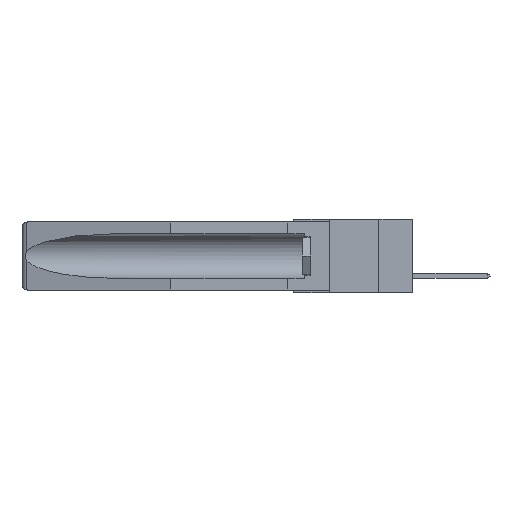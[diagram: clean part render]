
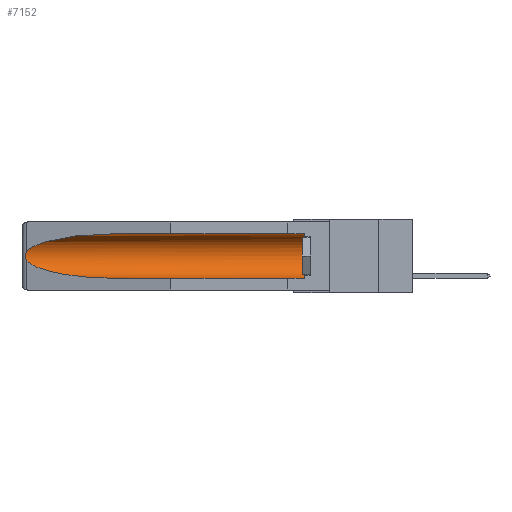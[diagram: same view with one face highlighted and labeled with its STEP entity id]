
A CAD part, left-side view. The second image highlights one B-rep face of the part: STEP entity #7152.
In plain terms, the highlighted cylindrical face has radius 2.857 mm (diameter 5.715 mm), a partial arc.
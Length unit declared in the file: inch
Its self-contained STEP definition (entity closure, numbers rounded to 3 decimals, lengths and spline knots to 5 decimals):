
#70 = CARTESIAN_POINT ( 'NONE',  ( 0.155, 1.07973, -0.284 ) ) ;
#157 = EDGE_CURVE ( 'NONE', #4583, #22965, #17708, .T. ) ;
#177 = B_SPLINE_CURVE_WITH_KNOTS ( 'NONE', 3,
 ( #16768, #13130, #5943, #20086, #11157, #260, #22140, #5716, #7740, #16540 ),
 .UNSPECIFIED., .F., .F.,
 ( 4, 2, 2, 2, 4 ),
 ( 0., 0.00029, 0.00058, 0.00087, 0.00117 ),
 .UNSPECIFIED. ) ;
#260 = CARTESIAN_POINT ( 'NONE',  ( 0.2675, 1.53308, -0.17534 ) ) ;
#667 = VERTEX_POINT ( 'NONE', #22013 ) ;
#1277 = AXIS2_PLACEMENT_3D ( 'NONE', #19700, #12644, #16241 ) ;
#1362 = CARTESIAN_POINT ( 'NONE',  ( 0.26537, 1.52718, -0.14972 ) ) ;
#3206 = ORIENTED_EDGE ( 'NONE', *, *, #15654, .T. ) ;
#3761 = FACE_OUTER_BOUND ( 'NONE', #9594, .T. ) ;
#4583 = VERTEX_POINT ( 'NONE', #7390 ) ;
#4636 = ORIENTED_EDGE ( 'NONE', *, *, #4979, .F. ) ;
#4810 = LINE ( 'NONE', #12451, #5923 ) ;
#4916 = ORIENTED_EDGE ( 'NONE', *, *, #11401, .T. ) ;
#4979 = EDGE_CURVE ( 'NONE', #4583, #667, #4810, .T. ) ;
#5716 = CARTESIAN_POINT ( 'NONE',  ( 0.26655, 1.53094, -0.18657 ) ) ;
#5923 = VECTOR ( 'NONE', #19657, 39.37008 ) ;
#5943 = CARTESIAN_POINT ( 'NONE',  ( 0.26654, 1.53092, -0.15636 ) ) ;
#7152 = ADVANCED_FACE ( 'NONE', ( #3761 ), #22407, .F. ) ;
#7186 = DIRECTION ( 'NONE',  ( 0., 1., 0. ) ) ;
#7390 = CARTESIAN_POINT ( 'NONE',  ( 0.155, 0.126, -0.284 ) ) ;
#7426 = CARTESIAN_POINT ( 'NONE',  ( 0.155, -0.30754, -0.1715 ) ) ;
#7740 = CARTESIAN_POINT ( 'NONE',  ( 0.26597, 1.5296, -0.19026 ) ) ;
#7965 = AXIS2_PLACEMENT_3D ( 'NONE', #7426, #7186, #10779 ) ;
#8923 = CARTESIAN_POINT ( 'NONE',  ( 0.26537, 1.52718, -0.14972 ) ) ;
#8979 = CARTESIAN_POINT ( 'NONE',  ( 0.25451, 1.48313, -0.24835 ) ) ;
#9292 = ORIENTED_EDGE ( 'NONE', *, *, #157, .T. ) ;
#9594 = EDGE_LOOP ( 'NONE', ( #10527, #4916, #3206, #4636, #9292, #17891 ) ) ;
#9619 = VECTOR ( 'NONE', #18152, 39.37008 ) ;
#10002 = EDGE_CURVE ( 'NONE', #22965, #20564, #22347, .T. ) ;
#10527 = ORIENTED_EDGE ( 'NONE', *, *, #13786, .T. ) ;
#10779 = DIRECTION ( 'NONE',  ( 0., 0., 1. ) ) ;
#11037 =( BOUNDED_CURVE ( )  B_SPLINE_CURVE ( 3, ( #14001, #11938, #17457, #1362 ),
 .UNSPECIFIED., .F., .F. ) 
 B_SPLINE_CURVE_WITH_KNOTS ( ( 4, 4 ),
 ( 4.71239, 6.08839 ),
 .UNSPECIFIED. ) 
 CURVE ( )  GEOMETRIC_REPRESENTATION_ITEM ( )  RATIONAL_B_SPLINE_CURVE ( ( 1., 0.848, 0.848, 1. ) ) 
 REPRESENTATION_ITEM ( '' )  );
#11157 = CARTESIAN_POINT ( 'NONE',  ( 0.2675, 1.53308, -0.16763 ) ) ;
#11209 = CARTESIAN_POINT ( 'NONE',  ( 0.155, 0.126, -0.059 ) ) ;
#11401 = EDGE_CURVE ( 'NONE', #13342, #14690, #177, .T. ) ;
#11761 =( BOUNDED_CURVE ( )  B_SPLINE_CURVE ( 3, ( #14393, #8979, #21698, #70 ),
 .UNSPECIFIED., .F., .F. ) 
 B_SPLINE_CURVE_WITH_KNOTS ( ( 4, 4 ),
 ( 0.1948, 1.5708 ),
 .UNSPECIFIED. ) 
 CURVE ( )  GEOMETRIC_REPRESENTATION_ITEM ( )  RATIONAL_B_SPLINE_CURVE ( ( 1., 0.848, 0.848, 1. ) ) 
 REPRESENTATION_ITEM ( '' )  );
#11938 = CARTESIAN_POINT ( 'NONE',  ( 0.21114, 1.30732, -0.059 ) ) ;
#12451 = CARTESIAN_POINT ( 'NONE',  ( 0.155, -0.30754, -0.284 ) ) ;
#12644 = DIRECTION ( 'NONE',  ( 0., -1., 0. ) ) ;
#13130 = CARTESIAN_POINT ( 'NONE',  ( 0.26597, 1.52961, -0.15275 ) ) ;
#13342 = VERTEX_POINT ( 'NONE', #8923 ) ;
#13786 = EDGE_CURVE ( 'NONE', #20564, #13342, #11037, .T. ) ;
#14001 = CARTESIAN_POINT ( 'NONE',  ( 0.155, 1.07973, -0.059 ) ) ;
#14393 = CARTESIAN_POINT ( 'NONE',  ( 0.26537, 1.52718, -0.19328 ) ) ;
#14690 = VERTEX_POINT ( 'NONE', #22626 ) ;
#15654 = EDGE_CURVE ( 'NONE', #14690, #667, #11761, .T. ) ;
#16241 = DIRECTION ( 'NONE',  ( 0., 0., 1. ) ) ;
#16540 = CARTESIAN_POINT ( 'NONE',  ( 0.26537, 1.52718, -0.19328 ) ) ;
#16768 = CARTESIAN_POINT ( 'NONE',  ( 0.26537, 1.52718, -0.14972 ) ) ;
#17457 = CARTESIAN_POINT ( 'NONE',  ( 0.25451, 1.48313, -0.09465 ) ) ;
#17708 = CIRCLE ( 'NONE', #1277, 0.1125 ) ;
#17891 = ORIENTED_EDGE ( 'NONE', *, *, #10002, .T. ) ;
#18152 = DIRECTION ( 'NONE',  ( 0., 1., 0. ) ) ;
#19657 = DIRECTION ( 'NONE',  ( 0., 1., 0. ) ) ;
#19700 = CARTESIAN_POINT ( 'NONE',  ( 0.155, 0.126, -0.1715 ) ) ;
#19724 = CARTESIAN_POINT ( 'NONE',  ( 0.155, -0.30754, -0.059 ) ) ;
#20086 = CARTESIAN_POINT ( 'NONE',  ( 0.2673, 1.5327, -0.16383 ) ) ;
#20564 = VERTEX_POINT ( 'NONE', #23271 ) ;
#21698 = CARTESIAN_POINT ( 'NONE',  ( 0.21114, 1.30732, -0.284 ) ) ;
#22013 = CARTESIAN_POINT ( 'NONE',  ( 0.155, 1.07973, -0.284 ) ) ;
#22140 = CARTESIAN_POINT ( 'NONE',  ( 0.2673, 1.53269, -0.17917 ) ) ;
#22347 = LINE ( 'NONE', #19724, #9619 ) ;
#22407 = CYLINDRICAL_SURFACE ( 'NONE', #7965, 0.1125 ) ;
#22626 = CARTESIAN_POINT ( 'NONE',  ( 0.26537, 1.52718, -0.19328 ) ) ;
#22965 = VERTEX_POINT ( 'NONE', #11209 ) ;
#23271 = CARTESIAN_POINT ( 'NONE',  ( 0.155, 1.07973, -0.059 ) ) ;
